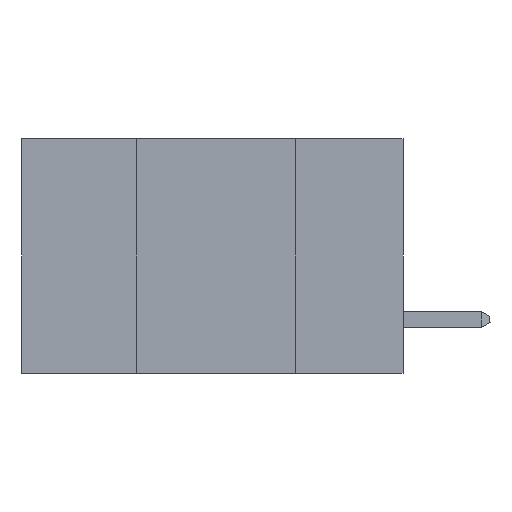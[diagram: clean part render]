
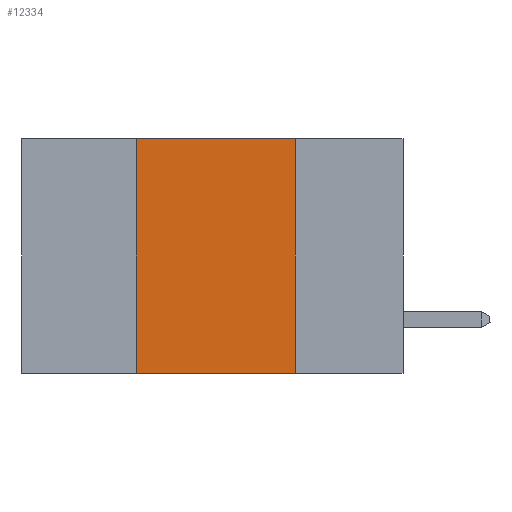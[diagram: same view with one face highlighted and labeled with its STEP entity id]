
A CAD part, left-side view. The second image highlights one B-rep face of the part: STEP entity #12334.
In plain terms, the highlighted planar face has unit normal (-1, 0, 0).
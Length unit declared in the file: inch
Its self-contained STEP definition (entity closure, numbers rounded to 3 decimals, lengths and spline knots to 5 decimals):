
#547 = PLANE ( 'NONE',  #12393 ) ;
#1285 = DIRECTION ( 'NONE',  ( 0., 0., -1. ) ) ;
#4261 = ORIENTED_EDGE ( 'NONE', *, *, #21301, .F. ) ;
#4586 = LINE ( 'NONE', #20681, #27167 ) ;
#6019 = EDGE_CURVE ( 'NONE', #37213, #11234, #39631, .T. ) ;
#6965 = VECTOR ( 'NONE', #26905, 39.37008 ) ;
#7574 = VECTOR ( 'NONE', #1285, 39.37008 ) ;
#9565 = EDGE_CURVE ( 'NONE', #18469, #11234, #33553, .T. ) ;
#9679 = EDGE_LOOP ( 'NONE', ( #27447, #4261, #24387, #25006 ) ) ;
#10447 = EDGE_CURVE ( 'NONE', #18469, #28216, #4586, .T. ) ;
#11056 = DIRECTION ( 'NONE',  ( 0., 0., -1. ) ) ;
#11209 = CARTESIAN_POINT ( 'NONE',  ( 0., 0.17, 0. ) ) ;
#11234 = VERTEX_POINT ( 'NONE', #21970 ) ;
#12334 = ADVANCED_FACE ( 'NONE', ( #29743 ), #547, .F. ) ;
#12393 = AXIS2_PLACEMENT_3D ( 'NONE', #27374, #27519, #11056 ) ;
#13125 = VECTOR ( 'NONE', #34333, 39.37008 ) ;
#18469 = VERTEX_POINT ( 'NONE', #32887 ) ;
#18564 = CARTESIAN_POINT ( 'NONE',  ( 0., 0.17, 0. ) ) ;
#20681 = CARTESIAN_POINT ( 'NONE',  ( 0., 0.42, 0. ) ) ;
#21301 = EDGE_CURVE ( 'NONE', #28216, #37213, #27998, .T. ) ;
#21970 = CARTESIAN_POINT ( 'NONE',  ( 0., 0.17, -0.37 ) ) ;
#24387 = ORIENTED_EDGE ( 'NONE', *, *, #10447, .F. ) ;
#25006 = ORIENTED_EDGE ( 'NONE', *, *, #9565, .T. ) ;
#26905 = DIRECTION ( 'NONE',  ( 0., -1., 0. ) ) ;
#27167 = VECTOR ( 'NONE', #41357, 39.37008 ) ;
#27374 = CARTESIAN_POINT ( 'NONE',  ( 0., 0.6, 0. ) ) ;
#27447 = ORIENTED_EDGE ( 'NONE', *, *, #6019, .F. ) ;
#27519 = DIRECTION ( 'NONE',  ( 1., 0., 0. ) ) ;
#27998 = LINE ( 'NONE', #37321, #6965 ) ;
#28216 = VERTEX_POINT ( 'NONE', #32709 ) ;
#29743 = FACE_OUTER_BOUND ( 'NONE', #9679, .T. ) ;
#32709 = CARTESIAN_POINT ( 'NONE',  ( 0., 0.42, 0. ) ) ;
#32887 = CARTESIAN_POINT ( 'NONE',  ( 0., 0.42, -0.37 ) ) ;
#33553 = LINE ( 'NONE', #37574, #13125 ) ;
#34333 = DIRECTION ( 'NONE',  ( 0., -1., 0. ) ) ;
#37213 = VERTEX_POINT ( 'NONE', #18564 ) ;
#37321 = CARTESIAN_POINT ( 'NONE',  ( 0., 0.6, 0. ) ) ;
#37574 = CARTESIAN_POINT ( 'NONE',  ( 0., 0.6, -0.37 ) ) ;
#39631 = LINE ( 'NONE', #11209, #7574 ) ;
#41357 = DIRECTION ( 'NONE',  ( 0., 0., 1. ) ) ;
